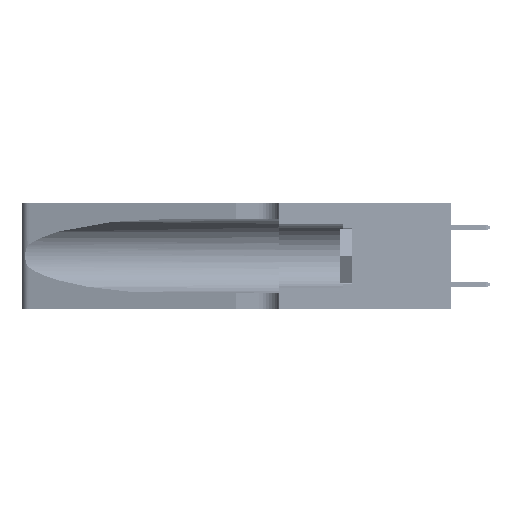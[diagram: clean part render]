
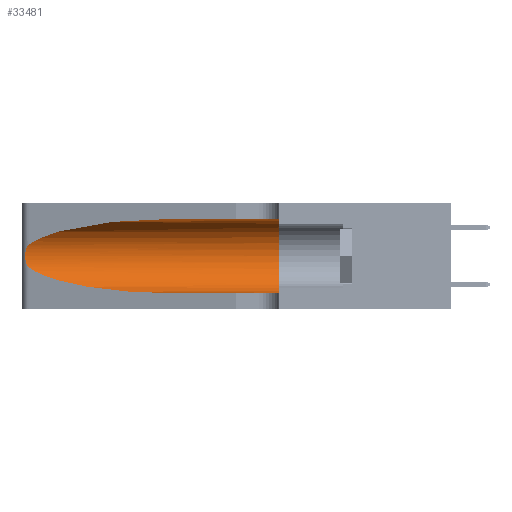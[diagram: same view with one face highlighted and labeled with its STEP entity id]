
A CAD part, left-side view. The second image highlights one B-rep face of the part: STEP entity #33481.
In plain terms, the highlighted cylindrical face has radius 3.308 mm (diameter 6.617 mm), a partial arc.
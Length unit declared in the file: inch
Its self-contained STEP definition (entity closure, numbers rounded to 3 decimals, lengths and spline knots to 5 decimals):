
#995 = CARTESIAN_POINT ( 'NONE',  ( 0.18966, 0.96281, 0.31525 ) ) ;
#1076 = EDGE_LOOP ( 'NONE', ( #34352, #41034, #25025, #8974, #29085, #2699 ) ) ;
#1335 = LINE ( 'NONE', #27263, #49150 ) ;
#2482 = CARTESIAN_POINT ( 'NONE',  ( 0.25487, 1.22718, 0.22369 ) ) ;
#2699 = ORIENTED_EDGE ( 'NONE', *, *, #11673, .F. ) ;
#2712 = LINE ( 'NONE', #15411, #19680 ) ;
#4237 = VERTEX_POINT ( 'NONE', #45916 ) ;
#4263 = CARTESIAN_POINT ( 'NONE',  ( 0.26017, 1.23833, 0.17102 ) ) ;
#4537 = CARTESIAN_POINT ( 'NONE',  ( 0.26075, 1.23896, 0.19203 ) ) ;
#5053 = CARTESIAN_POINT ( 'NONE',  ( 0.25555, 1.22993, 0.14849 ) ) ;
#5934 = DIRECTION ( 'NONE',  ( 0., -1., 0. ) ) ;
#6773 = DIRECTION ( 'NONE',  ( 0., -1., 0. ) ) ;
#7000 = CARTESIAN_POINT ( 'NONE',  ( 0.1305, 0.35, 0.31525 ) ) ;
#8073 = CARTESIAN_POINT ( 'NONE',  ( 0.25555, 1.22994, 0.2215 ) ) ;
#8502 = DIRECTION ( 'NONE',  ( 0., 1., 0. ) ) ;
#8593 = CARTESIAN_POINT ( 'NONE',  ( 0.25787, 1.23484, 0.2124 ) ) ;
#8974 = ORIENTED_EDGE ( 'NONE', *, *, #29731, .T. ) ;
#8997 = EDGE_CURVE ( 'NONE', #23748, #14086, #38997, .T. ) ;
#9126 = CARTESIAN_POINT ( 'NONE',  ( 0.26075, 1.23896, 0.178 ) ) ;
#10331 = AXIS2_PLACEMENT_3D ( 'NONE', #43544, #51943, #31376 ) ;
#11289 = EDGE_CURVE ( 'NONE', #51012, #36650, #30040, .T. ) ;
#11364 = VERTEX_POINT ( 'NONE', #41214 ) ;
#11673 = EDGE_CURVE ( 'NONE', #4237, #51012, #1335, .T. ) ;
#12884 = CARTESIAN_POINT ( 'NONE',  ( 0.25789, 1.23486, 0.15765 ) ) ;
#13147 = CARTESIAN_POINT ( 'NONE',  ( 0.25639, 1.23184, 0.21858 ) ) ;
#14086 = VERTEX_POINT ( 'NONE', #47462 ) ;
#15411 = CARTESIAN_POINT ( 'NONE',  ( 0.1305, 1.61858, 0.05475 ) ) ;
#17472 = CARTESIAN_POINT ( 'NONE',  ( 0.25487, 1.22718, 0.14631 ) ) ;
#19680 = VECTOR ( 'NONE', #6773, 39.37008 ) ;
#20343 =( BOUNDED_CURVE ( )  B_SPLINE_CURVE ( 3, ( #33464, #995, #46687, #34529 ),
 .UNSPECIFIED., .F., .T. ) 
 B_SPLINE_CURVE_WITH_KNOTS ( ( 4, 4 ),
 ( 1.5708, 2.84003 ),
 .UNSPECIFIED. ) 
 CURVE ( )  GEOMETRIC_REPRESENTATION_ITEM ( )  RATIONAL_B_SPLINE_CURVE ( ( 1., 0.87, 0.87, 1. ) ) 
 REPRESENTATION_ITEM ( '' )  );
#22066 = B_SPLINE_CURVE_WITH_KNOTS ( 'NONE', 3,
 ( #2482, #8073, #13147, #8593, #29386, #25311, #4537, #9126, #4263, #49423, #12884, #45660, #5053, #17472 ),
 .UNSPECIFIED., .F., .F.,
 ( 4, 2, 2, 2, 2, 2, 4 ),
 ( 0., 0.00027, 0.00053, 0.00107, 0.0016, 0.00187, 0.00214 ),
 .UNSPECIFIED. ) ;
#22703 = FACE_OUTER_BOUND ( 'NONE', #1076, .T. ) ;
#23491 = EDGE_CURVE ( 'NONE', #11364, #23748, #22066, .T. ) ;
#23748 = VERTEX_POINT ( 'NONE', #52633 ) ;
#25025 = ORIENTED_EDGE ( 'NONE', *, *, #8997, .T. ) ;
#25311 = CARTESIAN_POINT ( 'NONE',  ( 0.26018, 1.23835, 0.19895 ) ) ;
#27263 = CARTESIAN_POINT ( 'NONE',  ( 0.1305, 1.61858, 0.31525 ) ) ;
#27289 = CYLINDRICAL_SURFACE ( 'NONE', #10331, 0.13025 ) ;
#28076 = CARTESIAN_POINT ( 'NONE',  ( 0.25487, 1.22718, 0.14631 ) ) ;
#28347 = CARTESIAN_POINT ( 'NONE',  ( 0.18966, 0.96281, 0.05475 ) ) ;
#29085 = ORIENTED_EDGE ( 'NONE', *, *, #11289, .F. ) ;
#29386 = CARTESIAN_POINT ( 'NONE',  ( 0.25854, 1.2359, 0.20912 ) ) ;
#29731 = EDGE_CURVE ( 'NONE', #14086, #36650, #2712, .T. ) ;
#30040 = CIRCLE ( 'NONE', #31818, 0.13025 ) ;
#31376 = DIRECTION ( 'NONE',  ( 0., 0., -1. ) ) ;
#31635 = CARTESIAN_POINT ( 'NONE',  ( 0.1305, 0.72297, 0.05475 ) ) ;
#31818 = AXIS2_PLACEMENT_3D ( 'NONE', #33369, #8502, #40686 ) ;
#33369 = CARTESIAN_POINT ( 'NONE',  ( 0.1305, 0.35, 0.185 ) ) ;
#33464 = CARTESIAN_POINT ( 'NONE',  ( 0.1305, 0.72297, 0.31525 ) ) ;
#33465 = CARTESIAN_POINT ( 'NONE',  ( 0.1305, 0.35, 0.05475 ) ) ;
#33481 = ADVANCED_FACE ( 'NONE', ( #22703 ), #27289, .F. ) ;
#34352 = ORIENTED_EDGE ( 'NONE', *, *, #48430, .T. ) ;
#34529 = CARTESIAN_POINT ( 'NONE',  ( 0.25487, 1.22718, 0.22369 ) ) ;
#35963 = CARTESIAN_POINT ( 'NONE',  ( 0.2373, 1.15595, 0.08982 ) ) ;
#36650 = VERTEX_POINT ( 'NONE', #33465 ) ;
#38997 =( BOUNDED_CURVE ( )  B_SPLINE_CURVE ( 3, ( #28076, #35963, #28347, #31635 ),
 .UNSPECIFIED., .F., .F. ) 
 B_SPLINE_CURVE_WITH_KNOTS ( ( 4, 4 ),
 ( 3.44316, 4.71239 ),
 .UNSPECIFIED. ) 
 CURVE ( )  GEOMETRIC_REPRESENTATION_ITEM ( )  RATIONAL_B_SPLINE_CURVE ( ( 1., 0.87, 0.87, 1. ) ) 
 REPRESENTATION_ITEM ( '' )  );
#40686 = DIRECTION ( 'NONE',  ( 0., 0., 1. ) ) ;
#41034 = ORIENTED_EDGE ( 'NONE', *, *, #23491, .T. ) ;
#41214 = CARTESIAN_POINT ( 'NONE',  ( 0.25487, 1.22718, 0.22369 ) ) ;
#43544 = CARTESIAN_POINT ( 'NONE',  ( 0.1305, 1.61858, 0.185 ) ) ;
#45660 = CARTESIAN_POINT ( 'NONE',  ( 0.25639, 1.23186, 0.15144 ) ) ;
#45916 = CARTESIAN_POINT ( 'NONE',  ( 0.1305, 0.72297, 0.31525 ) ) ;
#46687 = CARTESIAN_POINT ( 'NONE',  ( 0.2373, 1.15595, 0.28018 ) ) ;
#47462 = CARTESIAN_POINT ( 'NONE',  ( 0.1305, 0.72297, 0.05475 ) ) ;
#48430 = EDGE_CURVE ( 'NONE', #4237, #11364, #20343, .T. ) ;
#49150 = VECTOR ( 'NONE', #5934, 39.37008 ) ;
#49423 = CARTESIAN_POINT ( 'NONE',  ( 0.25856, 1.23593, 0.16098 ) ) ;
#51012 = VERTEX_POINT ( 'NONE', #7000 ) ;
#51943 = DIRECTION ( 'NONE',  ( 0., -1., 0. ) ) ;
#52633 = CARTESIAN_POINT ( 'NONE',  ( 0.25487, 1.22718, 0.14631 ) ) ;
